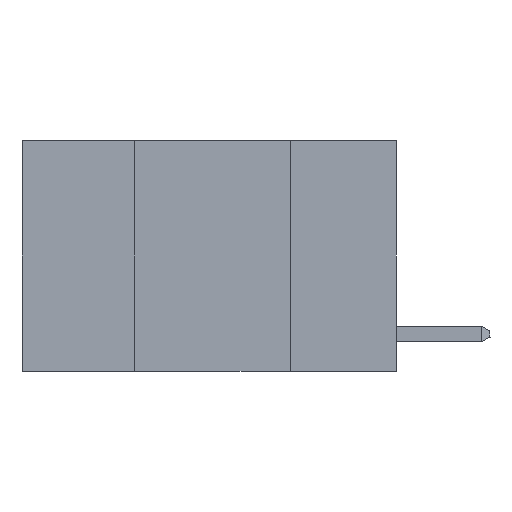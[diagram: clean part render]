
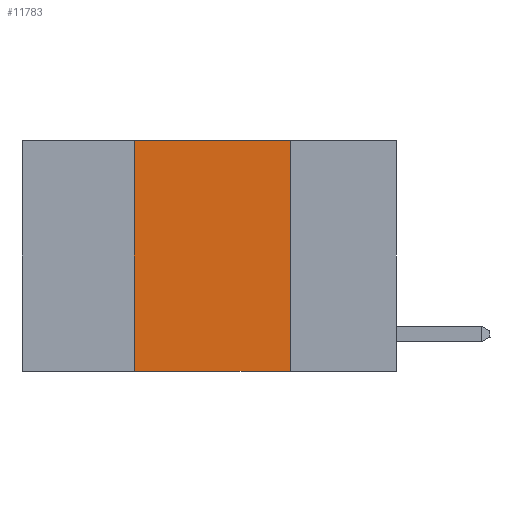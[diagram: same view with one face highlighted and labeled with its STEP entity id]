
A CAD part, left-side view. The second image highlights one B-rep face of the part: STEP entity #11783.
In plain terms, the highlighted planar face has unit normal (-1, 0, 0).
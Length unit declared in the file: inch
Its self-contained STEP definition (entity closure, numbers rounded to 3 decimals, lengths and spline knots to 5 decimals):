
#3022 = LINE ( 'NONE', #11641, #14679 ) ;
#3184 = CARTESIAN_POINT ( 'NONE',  ( 0., 0.42, 0. ) ) ;
#4000 = CARTESIAN_POINT ( 'NONE',  ( 0., 0.6, -0.37 ) ) ;
#4098 = ORIENTED_EDGE ( 'NONE', *, *, #10201, .F. ) ;
#4768 = ORIENTED_EDGE ( 'NONE', *, *, #11945, .T. ) ;
#5196 = CARTESIAN_POINT ( 'NONE',  ( 0., 0.6, 0. ) ) ;
#5494 = EDGE_CURVE ( 'NONE', #10300, #11720, #3022, .T. ) ;
#6639 = EDGE_CURVE ( 'NONE', #7238, #10300, #11693, .T. ) ;
#6785 = AXIS2_PLACEMENT_3D ( 'NONE', #5196, #8378, #19355 ) ;
#6802 = PLANE ( 'NONE',  #6785 ) ;
#6922 = DIRECTION ( 'NONE',  ( 0., -1., 0. ) ) ;
#7238 = VERTEX_POINT ( 'NONE', #16346 ) ;
#7474 = VECTOR ( 'NONE', #20531, 39.37008 ) ;
#8378 = DIRECTION ( 'NONE',  ( 1., 0., 0. ) ) ;
#9196 = ORIENTED_EDGE ( 'NONE', *, *, #5494, .F. ) ;
#9379 = DIRECTION ( 'NONE',  ( 0., 0., -1. ) ) ;
#9514 = FACE_OUTER_BOUND ( 'NONE', #20408, .T. ) ;
#10201 = EDGE_CURVE ( 'NONE', #11720, #10439, #16662, .T. ) ;
#10300 = VERTEX_POINT ( 'NONE', #15610 ) ;
#10439 = VERTEX_POINT ( 'NONE', #19065 ) ;
#10725 = VECTOR ( 'NONE', #15077, 39.37008 ) ;
#10963 = CARTESIAN_POINT ( 'NONE',  ( 0., 0.17, 0. ) ) ;
#11641 = CARTESIAN_POINT ( 'NONE',  ( 0., 0.6, 0. ) ) ;
#11693 = LINE ( 'NONE', #3184, #7474 ) ;
#11720 = VERTEX_POINT ( 'NONE', #14526 ) ;
#11783 = ADVANCED_FACE ( 'NONE', ( #9514 ), #6802, .F. ) ;
#11945 = EDGE_CURVE ( 'NONE', #7238, #10439, #14412, .T. ) ;
#12993 = VECTOR ( 'NONE', #9379, 39.37008 ) ;
#13187 = ORIENTED_EDGE ( 'NONE', *, *, #6639, .F. ) ;
#14412 = LINE ( 'NONE', #4000, #10725 ) ;
#14526 = CARTESIAN_POINT ( 'NONE',  ( 0., 0.17, 0. ) ) ;
#14679 = VECTOR ( 'NONE', #6922, 39.37008 ) ;
#15077 = DIRECTION ( 'NONE',  ( 0., -1., 0. ) ) ;
#15610 = CARTESIAN_POINT ( 'NONE',  ( 0., 0.42, 0. ) ) ;
#16346 = CARTESIAN_POINT ( 'NONE',  ( 0., 0.42, -0.37 ) ) ;
#16662 = LINE ( 'NONE', #10963, #12993 ) ;
#19065 = CARTESIAN_POINT ( 'NONE',  ( 0., 0.17, -0.37 ) ) ;
#19355 = DIRECTION ( 'NONE',  ( 0., 0., -1. ) ) ;
#20408 = EDGE_LOOP ( 'NONE', ( #4098, #9196, #13187, #4768 ) ) ;
#20531 = DIRECTION ( 'NONE',  ( 0., 0., 1. ) ) ;
